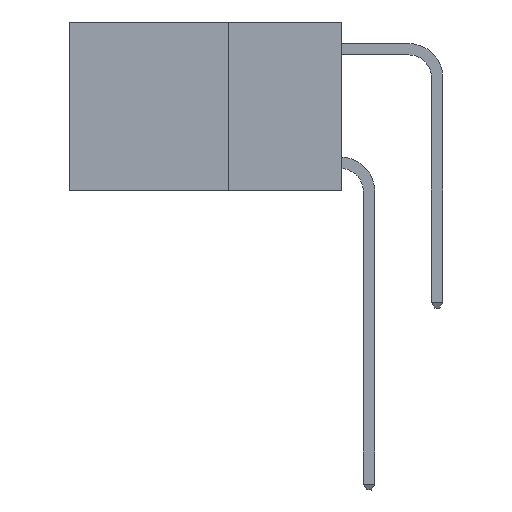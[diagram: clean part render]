
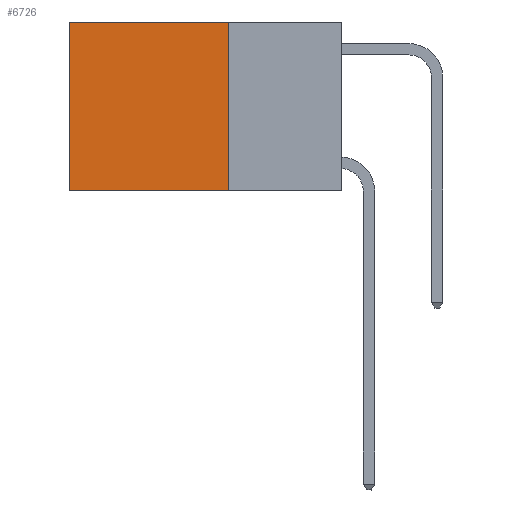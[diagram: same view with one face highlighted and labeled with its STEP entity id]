
A CAD part, left-side view. The second image highlights one B-rep face of the part: STEP entity #6726.
In plain terms, the highlighted planar face has unit normal (-1, 0, 0).
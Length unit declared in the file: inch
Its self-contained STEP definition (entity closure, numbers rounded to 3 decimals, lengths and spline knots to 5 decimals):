
#1570 = EDGE_CURVE ( 'NONE', #10449, #26204, #14160, .T. ) ;
#2608 = CARTESIAN_POINT ( 'NONE',  ( 0.2625, 0.6, -0.37 ) ) ;
#2705 = ORIENTED_EDGE ( 'NONE', *, *, #15432, .F. ) ;
#3917 = ORIENTED_EDGE ( 'NONE', *, *, #20345, .T. ) ;
#4200 = DIRECTION ( 'NONE',  ( 1., 0., 0. ) ) ;
#5194 = DIRECTION ( 'NONE',  ( 0., 1., 0. ) ) ;
#5451 = AXIS2_PLACEMENT_3D ( 'NONE', #16269, #4200, #25904 ) ;
#6726 = ADVANCED_FACE ( 'NONE', ( #23183 ), #16114, .F. ) ;
#9215 = DIRECTION ( 'NONE',  ( 0., 1., 0. ) ) ;
#9530 = CARTESIAN_POINT ( 'NONE',  ( 0.2625, 0.25, -0.37 ) ) ;
#10103 = EDGE_CURVE ( 'NONE', #21899, #17171, #24732, .T. ) ;
#10449 = VERTEX_POINT ( 'NONE', #18584 ) ;
#10668 = CARTESIAN_POINT ( 'NONE',  ( 0.2625, 0.6, 0. ) ) ;
#12033 = DIRECTION ( 'NONE',  ( 0., 0., -1. ) ) ;
#12603 = LINE ( 'NONE', #9530, #29920 ) ;
#14160 = LINE ( 'NONE', #23813, #29073 ) ;
#14799 = ORIENTED_EDGE ( 'NONE', *, *, #10103, .T. ) ;
#14804 = EDGE_LOOP ( 'NONE', ( #14799, #2705, #28819, #3917 ) ) ;
#15432 = EDGE_CURVE ( 'NONE', #26204, #17171, #12603, .T. ) ;
#16114 = PLANE ( 'NONE',  #5451 ) ;
#16269 = CARTESIAN_POINT ( 'NONE',  ( 0.2625, 0.25, 0. ) ) ;
#17016 = CARTESIAN_POINT ( 'NONE',  ( 0.2625, 0.6, 0. ) ) ;
#17171 = VERTEX_POINT ( 'NONE', #2608 ) ;
#18584 = CARTESIAN_POINT ( 'NONE',  ( 0.2625, 0.25, 0. ) ) ;
#19126 = DIRECTION ( 'NONE',  ( 0., 0., -1. ) ) ;
#20345 = EDGE_CURVE ( 'NONE', #10449, #21899, #24330, .T. ) ;
#20457 = VECTOR ( 'NONE', #12033, 39.37008 ) ;
#21899 = VERTEX_POINT ( 'NONE', #10668 ) ;
#23183 = FACE_OUTER_BOUND ( 'NONE', #14804, .T. ) ;
#23813 = CARTESIAN_POINT ( 'NONE',  ( 0.2625, 0.25, 0. ) ) ;
#24330 = LINE ( 'NONE', #28834, #28074 ) ;
#24732 = LINE ( 'NONE', #17016, #20457 ) ;
#25904 = DIRECTION ( 'NONE',  ( 0., 0., -1. ) ) ;
#26204 = VERTEX_POINT ( 'NONE', #26468 ) ;
#26468 = CARTESIAN_POINT ( 'NONE',  ( 0.2625, 0.25, -0.37 ) ) ;
#28074 = VECTOR ( 'NONE', #9215, 39.37008 ) ;
#28819 = ORIENTED_EDGE ( 'NONE', *, *, #1570, .F. ) ;
#28834 = CARTESIAN_POINT ( 'NONE',  ( 0.2625, 0.25, 0. ) ) ;
#29073 = VECTOR ( 'NONE', #19126, 39.37008 ) ;
#29920 = VECTOR ( 'NONE', #5194, 39.37008 ) ;
